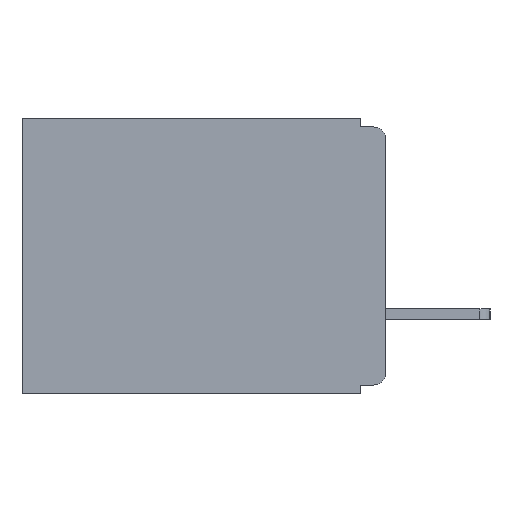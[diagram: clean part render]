
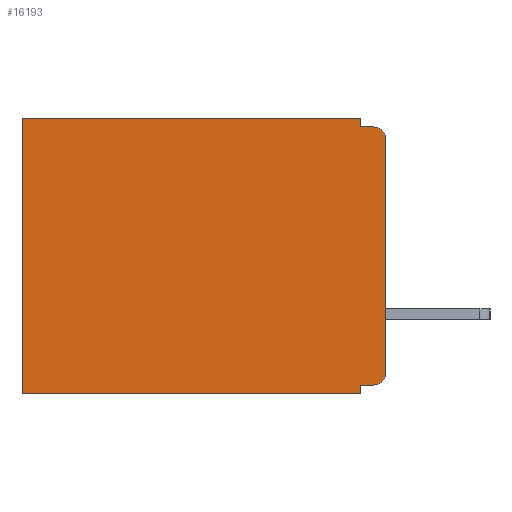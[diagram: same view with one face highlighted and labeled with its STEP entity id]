
A CAD part, left-side view. The second image highlights one B-rep face of the part: STEP entity #16193.
In plain terms, the highlighted planar face has unit normal (-1, 0, 0).
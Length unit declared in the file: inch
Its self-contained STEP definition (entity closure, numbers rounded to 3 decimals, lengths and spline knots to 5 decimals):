
#337 = FACE_OUTER_BOUND ( 'NONE', #18190, .T. ) ;
#580 = CARTESIAN_POINT ( 'NONE',  ( 0.3, 0.031, -0.32 ) ) ;
#838 = DIRECTION ( 'NONE',  ( 0., 0., -1. ) ) ;
#2709 = CARTESIAN_POINT ( 'NONE',  ( 0.3, 0., -0.025 ) ) ;
#3119 = CARTESIAN_POINT ( 'NONE',  ( 0.3, 0., -0.33 ) ) ;
#3228 = LINE ( 'NONE', #11252, #27516 ) ;
#3416 = VERTEX_POINT ( 'NONE', #24667 ) ;
#3562 = ORIENTED_EDGE ( 'NONE', *, *, #18641, .T. ) ;
#4017 = DIRECTION ( 'NONE',  ( 0., 0., -1. ) ) ;
#4127 = CARTESIAN_POINT ( 'NONE',  ( 0.3, 0.437, -0.33 ) ) ;
#4217 = EDGE_CURVE ( 'NONE', #21619, #16782, #3228, .T. ) ;
#4456 = CARTESIAN_POINT ( 'NONE',  ( 0.3, 0., 0. ) ) ;
#4769 = VERTEX_POINT ( 'NONE', #26028 ) ;
#5271 = VECTOR ( 'NONE', #4017, 39.37008 ) ;
#5336 = CARTESIAN_POINT ( 'NONE',  ( 0.3, 0.015, -0.305 ) ) ;
#5768 = LINE ( 'NONE', #26126, #23884 ) ;
#5867 = DIRECTION ( 'NONE',  ( 0., 0., -1. ) ) ;
#6230 = AXIS2_PLACEMENT_3D ( 'NONE', #5336, #21928, #7729 ) ;
#6688 = DIRECTION ( 'NONE',  ( 0., 1., 0. ) ) ;
#6982 = VECTOR ( 'NONE', #29048, 39.37008 ) ;
#7729 = DIRECTION ( 'NONE',  ( 0., 0., -1. ) ) ;
#8981 = VECTOR ( 'NONE', #27886, 39.37008 ) ;
#9032 = AXIS2_PLACEMENT_3D ( 'NONE', #3119, #15156, #838 ) ;
#10568 = VERTEX_POINT ( 'NONE', #22930 ) ;
#11041 = DIRECTION ( 'NONE',  ( 0., 1., 0. ) ) ;
#11178 = EDGE_CURVE ( 'NONE', #28164, #10568, #30156, .T. ) ;
#11216 = LINE ( 'NONE', #23340, #11972 ) ;
#11252 = CARTESIAN_POINT ( 'NONE',  ( 0.3, 0., -0.32 ) ) ;
#11863 = EDGE_CURVE ( 'NONE', #3416, #23506, #5768, .T. ) ;
#11972 = VECTOR ( 'NONE', #6688, 39.37008 ) ;
#12567 = ORIENTED_EDGE ( 'NONE', *, *, #20082, .F. ) ;
#12747 = AXIS2_PLACEMENT_3D ( 'NONE', #14113, #30215, #16483 ) ;
#13762 = LINE ( 'NONE', #15255, #6982 ) ;
#14113 = CARTESIAN_POINT ( 'NONE',  ( 0.3, 0.015, -0.025 ) ) ;
#14661 = CARTESIAN_POINT ( 'NONE',  ( 0.3, 0.437, 0. ) ) ;
#14908 = CIRCLE ( 'NONE', #6230, 0.015 ) ;
#15156 = DIRECTION ( 'NONE',  ( 1., 0., 0. ) ) ;
#15193 = VERTEX_POINT ( 'NONE', #22405 ) ;
#15255 = CARTESIAN_POINT ( 'NONE',  ( 0.3, 0.031, 0. ) ) ;
#16193 = ADVANCED_FACE ( 'NONE', ( #337 ), #24399, .F. ) ;
#16483 = DIRECTION ( 'NONE',  ( 0., 0., -1. ) ) ;
#16781 = EDGE_CURVE ( 'NONE', #21619, #15193, #14908, .T. ) ;
#16782 = VERTEX_POINT ( 'NONE', #580 ) ;
#16819 = CARTESIAN_POINT ( 'NONE',  ( 0.3, 0.031, -0.33 ) ) ;
#17022 = ORIENTED_EDGE ( 'NONE', *, *, #4217, .F. ) ;
#17725 = ORIENTED_EDGE ( 'NONE', *, *, #11863, .F. ) ;
#18190 = EDGE_LOOP ( 'NONE', ( #18787, #3562, #17725, #23878, #21343, #30277, #12567, #27146, #17022, #29249 ) ) ;
#18604 = CARTESIAN_POINT ( 'NONE',  ( 0.3, 0., -0.33 ) ) ;
#18641 = EDGE_CURVE ( 'NONE', #18767, #23506, #28771, .T. ) ;
#18767 = VERTEX_POINT ( 'NONE', #2709 ) ;
#18787 = ORIENTED_EDGE ( 'NONE', *, *, #26769, .F. ) ;
#19033 = EDGE_CURVE ( 'NONE', #16782, #24278, #30142, .T. ) ;
#20082 = EDGE_CURVE ( 'NONE', #24278, #10568, #11216, .T. ) ;
#20107 = CARTESIAN_POINT ( 'NONE',  ( 0.3, 0.031, -0.33 ) ) ;
#21343 = ORIENTED_EDGE ( 'NONE', *, *, #21836, .T. ) ;
#21521 = EDGE_CURVE ( 'NONE', #4769, #3416, #13762, .T. ) ;
#21619 = VERTEX_POINT ( 'NONE', #22547 ) ;
#21836 = EDGE_CURVE ( 'NONE', #4769, #28164, #28615, .T. ) ;
#21928 = DIRECTION ( 'NONE',  ( -1., 0., 0. ) ) ;
#22405 = CARTESIAN_POINT ( 'NONE',  ( 0.3, 0., -0.305 ) ) ;
#22547 = CARTESIAN_POINT ( 'NONE',  ( 0.3, 0.015, -0.32 ) ) ;
#22661 = VECTOR ( 'NONE', #5867, 39.37008 ) ;
#22930 = CARTESIAN_POINT ( 'NONE',  ( 0.3, 0.437, -0.33 ) ) ;
#23008 = LINE ( 'NONE', #18604, #8981 ) ;
#23340 = CARTESIAN_POINT ( 'NONE',  ( 0.3, 0., -0.33 ) ) ;
#23348 = DIRECTION ( 'NONE',  ( 0., 1., 0. ) ) ;
#23506 = VERTEX_POINT ( 'NONE', #30000 ) ;
#23878 = ORIENTED_EDGE ( 'NONE', *, *, #21521, .F. ) ;
#23884 = VECTOR ( 'NONE', #28398, 39.37008 ) ;
#24278 = VERTEX_POINT ( 'NONE', #16819 ) ;
#24399 = PLANE ( 'NONE',  #9032 ) ;
#24667 = CARTESIAN_POINT ( 'NONE',  ( 0.3, 0.031, -0.01 ) ) ;
#26028 = CARTESIAN_POINT ( 'NONE',  ( 0.3, 0.031, 0. ) ) ;
#26126 = CARTESIAN_POINT ( 'NONE',  ( 0.3, 0., -0.01 ) ) ;
#26769 = EDGE_CURVE ( 'NONE', #18767, #15193, #23008, .T. ) ;
#27146 = ORIENTED_EDGE ( 'NONE', *, *, #19033, .F. ) ;
#27516 = VECTOR ( 'NONE', #11041, 39.37008 ) ;
#27886 = DIRECTION ( 'NONE',  ( 0., 0., -1. ) ) ;
#27919 = VECTOR ( 'NONE', #23348, 39.37008 ) ;
#28164 = VERTEX_POINT ( 'NONE', #14661 ) ;
#28398 = DIRECTION ( 'NONE',  ( 0., -1., 0. ) ) ;
#28615 = LINE ( 'NONE', #4456, #27919 ) ;
#28771 = CIRCLE ( 'NONE', #12747, 0.015 ) ;
#29048 = DIRECTION ( 'NONE',  ( 0., 0., -1. ) ) ;
#29249 = ORIENTED_EDGE ( 'NONE', *, *, #16781, .T. ) ;
#30000 = CARTESIAN_POINT ( 'NONE',  ( 0.3, 0.015, -0.01 ) ) ;
#30142 = LINE ( 'NONE', #20107, #22661 ) ;
#30156 = LINE ( 'NONE', #4127, #5271 ) ;
#30215 = DIRECTION ( 'NONE',  ( -1., 0., 0. ) ) ;
#30277 = ORIENTED_EDGE ( 'NONE', *, *, #11178, .T. ) ;
